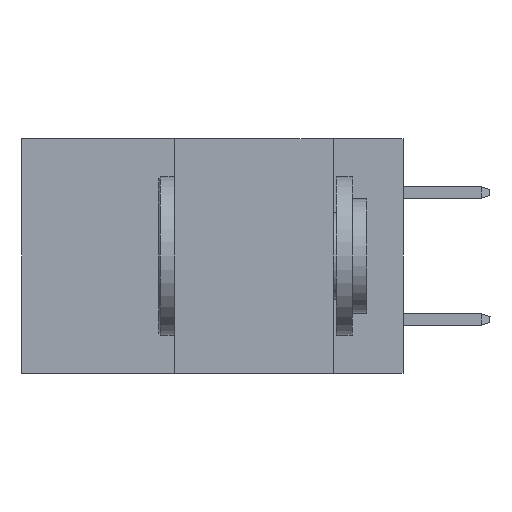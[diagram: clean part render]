
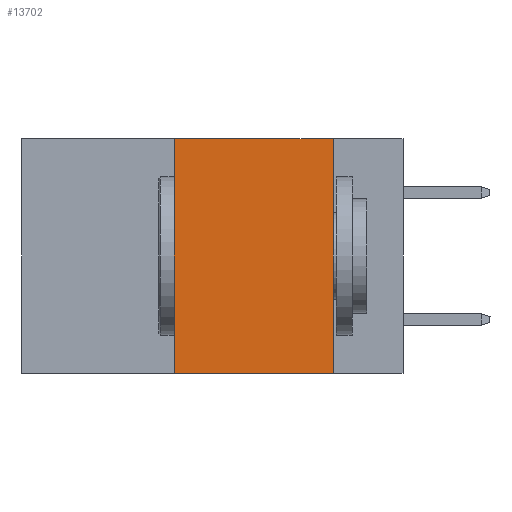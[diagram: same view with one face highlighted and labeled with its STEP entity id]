
A CAD part, left-side view. The second image highlights one B-rep face of the part: STEP entity #13702.
In plain terms, the highlighted planar face has unit normal (-1, 0, 0).
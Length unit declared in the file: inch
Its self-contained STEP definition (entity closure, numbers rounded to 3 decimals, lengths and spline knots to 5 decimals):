
#916 = VECTOR ( 'NONE', #23535, 39.37008 ) ;
#3542 = DIRECTION ( 'NONE',  ( 0., 0., 1. ) ) ;
#5707 = CARTESIAN_POINT ( 'NONE',  ( 0., 0.36, 0. ) ) ;
#6307 = VERTEX_POINT ( 'NONE', #18863 ) ;
#7194 = LINE ( 'NONE', #9475, #916 ) ;
#7570 = LINE ( 'NONE', #5707, #9500 ) ;
#7704 = ORIENTED_EDGE ( 'NONE', *, *, #26036, .F. ) ;
#7796 = ORIENTED_EDGE ( 'NONE', *, *, #9823, .T. ) ;
#8160 = CARTESIAN_POINT ( 'NONE',  ( 0., 0.6, 0. ) ) ;
#8477 = VECTOR ( 'NONE', #14650, 39.37008 ) ;
#8557 = LINE ( 'NONE', #12727, #8477 ) ;
#9094 = CARTESIAN_POINT ( 'NONE',  ( 0., 0.6, 0. ) ) ;
#9475 = CARTESIAN_POINT ( 'NONE',  ( 0., 0.11, 0. ) ) ;
#9500 = VECTOR ( 'NONE', #3542, 39.37008 ) ;
#9823 = EDGE_CURVE ( 'NONE', #24150, #24779, #8557, .T. ) ;
#10744 = EDGE_CURVE ( 'NONE', #6307, #12408, #12194, .T. ) ;
#11246 = DIRECTION ( 'NONE',  ( 0., 0., -1. ) ) ;
#12168 = ORIENTED_EDGE ( 'NONE', *, *, #10744, .F. ) ;
#12194 = LINE ( 'NONE', #8160, #17122 ) ;
#12408 = VERTEX_POINT ( 'NONE', #19620 ) ;
#12727 = CARTESIAN_POINT ( 'NONE',  ( 0., 0.6, -0.37 ) ) ;
#13079 = ORIENTED_EDGE ( 'NONE', *, *, #24161, .F. ) ;
#13702 = ADVANCED_FACE ( 'NONE', ( #15319 ), #25447, .F. ) ;
#14650 = DIRECTION ( 'NONE',  ( 0., -1., 0. ) ) ;
#15319 = FACE_OUTER_BOUND ( 'NONE', #22112, .T. ) ;
#17122 = VECTOR ( 'NONE', #19909, 39.37008 ) ;
#18863 = CARTESIAN_POINT ( 'NONE',  ( 0., 0.36, 0. ) ) ;
#19620 = CARTESIAN_POINT ( 'NONE',  ( 0., 0.11, 0. ) ) ;
#19732 = CARTESIAN_POINT ( 'NONE',  ( 0., 0.36, -0.37 ) ) ;
#19909 = DIRECTION ( 'NONE',  ( 0., -1., 0. ) ) ;
#21870 = CARTESIAN_POINT ( 'NONE',  ( 0., 0.11, -0.37 ) ) ;
#22112 = EDGE_LOOP ( 'NONE', ( #7704, #12168, #13079, #7796 ) ) ;
#23411 = DIRECTION ( 'NONE',  ( 1., 0., 0. ) ) ;
#23535 = DIRECTION ( 'NONE',  ( 0., 0., -1. ) ) ;
#24150 = VERTEX_POINT ( 'NONE', #19732 ) ;
#24161 = EDGE_CURVE ( 'NONE', #24150, #6307, #7570, .T. ) ;
#24779 = VERTEX_POINT ( 'NONE', #21870 ) ;
#25447 = PLANE ( 'NONE',  #25796 ) ;
#25796 = AXIS2_PLACEMENT_3D ( 'NONE', #9094, #23411, #11246 ) ;
#26036 = EDGE_CURVE ( 'NONE', #12408, #24779, #7194, .T. ) ;
